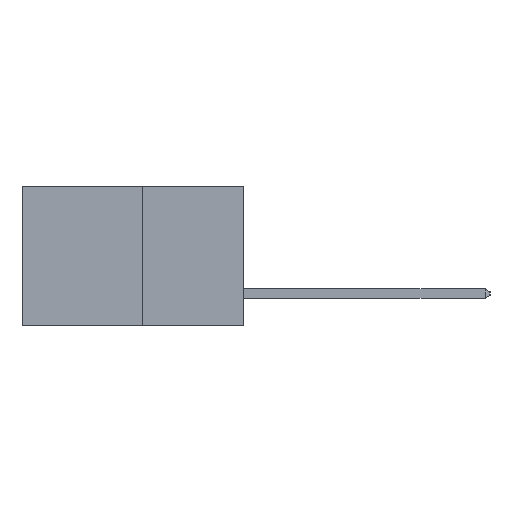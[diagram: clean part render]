
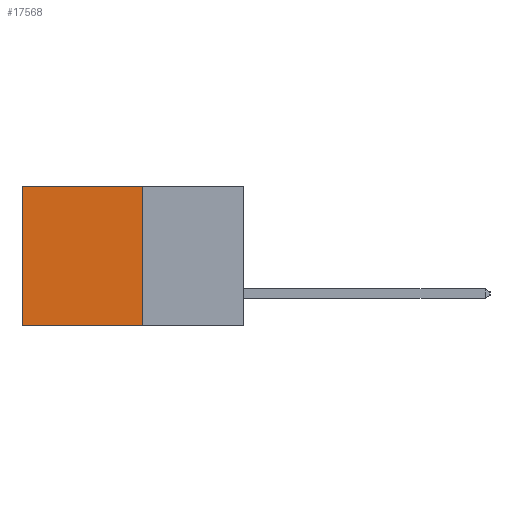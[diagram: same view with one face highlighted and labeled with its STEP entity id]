
A CAD part, left-side view. The second image highlights one B-rep face of the part: STEP entity #17568.
In plain terms, the highlighted planar face has unit normal (-1, 0, 0).
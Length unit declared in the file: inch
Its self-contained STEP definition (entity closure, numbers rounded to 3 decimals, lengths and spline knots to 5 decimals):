
#286 = CARTESIAN_POINT ( 'NONE',  ( 0.277, 0.59, 0. ) ) ;
#331 = DIRECTION ( 'NONE',  ( 0., 0., -1. ) ) ;
#478 = VECTOR ( 'NONE', #331, 39.37008 ) ;
#530 = DIRECTION ( 'NONE',  ( 1., 0., 0. ) ) ;
#3918 = CARTESIAN_POINT ( 'NONE',  ( 0.277, 0.27, -0.37 ) ) ;
#4237 = VECTOR ( 'NONE', #5883, 39.37008 ) ;
#4563 = CARTESIAN_POINT ( 'NONE',  ( 0.277, 0.27, -0.37 ) ) ;
#4775 = LINE ( 'NONE', #17896, #4237 ) ;
#5883 = DIRECTION ( 'NONE',  ( 0., 0., -1. ) ) ;
#6350 = ORIENTED_EDGE ( 'NONE', *, *, #6606, .F. ) ;
#6606 = EDGE_CURVE ( 'NONE', #19998, #11900, #18851, .T. ) ;
#8679 = VERTEX_POINT ( 'NONE', #9373 ) ;
#9154 = ORIENTED_EDGE ( 'NONE', *, *, #17015, .T. ) ;
#9373 = CARTESIAN_POINT ( 'NONE',  ( 0.277, 0.59, -0.37 ) ) ;
#10573 = AXIS2_PLACEMENT_3D ( 'NONE', #11010, #530, #12749 ) ;
#11010 = CARTESIAN_POINT ( 'NONE',  ( 0.277, 0.27, -0.37 ) ) ;
#11049 = LINE ( 'NONE', #4563, #20087 ) ;
#11900 = VERTEX_POINT ( 'NONE', #13763 ) ;
#12749 = DIRECTION ( 'NONE',  ( 0., 0., -1. ) ) ;
#13763 = CARTESIAN_POINT ( 'NONE',  ( 0.277, 0.27, -0.37 ) ) ;
#14447 = EDGE_CURVE ( 'NONE', #11900, #8679, #11049, .T. ) ;
#14945 = EDGE_CURVE ( 'NONE', #21503, #8679, #4775, .T. ) ;
#15815 = ORIENTED_EDGE ( 'NONE', *, *, #14447, .F. ) ;
#15926 = VECTOR ( 'NONE', #21493, 39.37008 ) ;
#17015 = EDGE_CURVE ( 'NONE', #19998, #21503, #20431, .T. ) ;
#17568 = ADVANCED_FACE ( 'NONE', ( #17725 ), #21192, .F. ) ;
#17725 = FACE_OUTER_BOUND ( 'NONE', #17771, .T. ) ;
#17771 = EDGE_LOOP ( 'NONE', ( #18173, #15815, #6350, #9154 ) ) ;
#17896 = CARTESIAN_POINT ( 'NONE',  ( 0.277, 0.59, -0.37 ) ) ;
#18173 = ORIENTED_EDGE ( 'NONE', *, *, #14945, .T. ) ;
#18217 = DIRECTION ( 'NONE',  ( 0., 1., 0. ) ) ;
#18851 = LINE ( 'NONE', #3918, #478 ) ;
#18926 = CARTESIAN_POINT ( 'NONE',  ( 0.277, 0.27, 0. ) ) ;
#19783 = CARTESIAN_POINT ( 'NONE',  ( 0.277, 0.27, 0. ) ) ;
#19998 = VERTEX_POINT ( 'NONE', #18926 ) ;
#20087 = VECTOR ( 'NONE', #18217, 39.37008 ) ;
#20431 = LINE ( 'NONE', #19783, #15926 ) ;
#21192 = PLANE ( 'NONE',  #10573 ) ;
#21493 = DIRECTION ( 'NONE',  ( 0., 1., 0. ) ) ;
#21503 = VERTEX_POINT ( 'NONE', #286 ) ;
